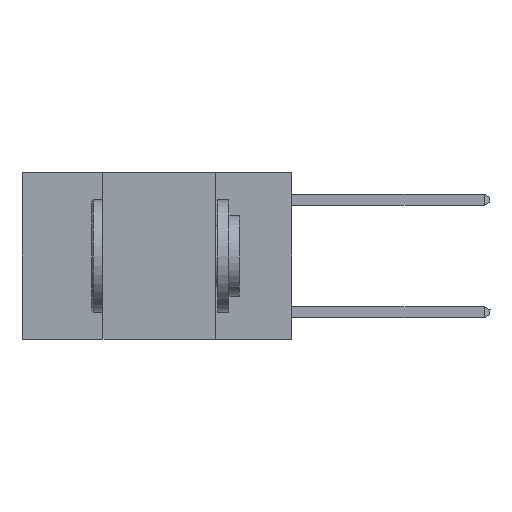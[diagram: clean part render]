
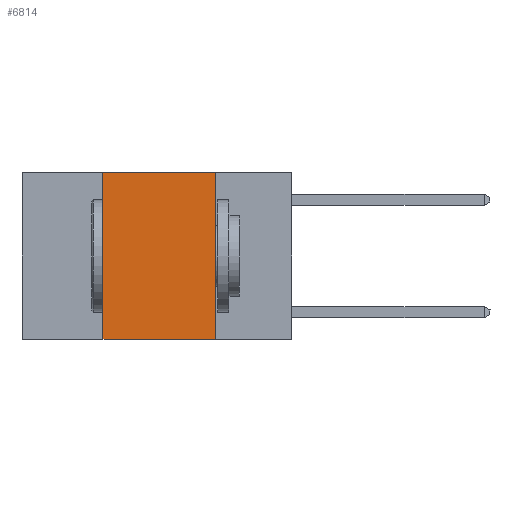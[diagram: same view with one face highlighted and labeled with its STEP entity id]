
A CAD part, left-side view. The second image highlights one B-rep face of the part: STEP entity #6814.
In plain terms, the highlighted planar face has unit normal (-1, 0, 0).
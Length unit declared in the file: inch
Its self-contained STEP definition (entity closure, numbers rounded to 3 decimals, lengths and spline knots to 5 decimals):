
#841 = VECTOR ( 'NONE', #13239, 39.37008 ) ;
#1133 = CARTESIAN_POINT ( 'NONE',  ( 0., 0.6, 0. ) ) ;
#1365 = DIRECTION ( 'NONE',  ( 0., 0., -1. ) ) ;
#2137 = CARTESIAN_POINT ( 'NONE',  ( 0., 0.42, -0.37 ) ) ;
#2207 = LINE ( 'NONE', #11647, #7037 ) ;
#3255 = DIRECTION ( 'NONE',  ( 1., 0., 0. ) ) ;
#4270 = LINE ( 'NONE', #20502, #19814 ) ;
#4390 = DIRECTION ( 'NONE',  ( 0., 0., 1. ) ) ;
#5343 = EDGE_CURVE ( 'NONE', #6308, #20521, #22432, .T. ) ;
#6036 = CARTESIAN_POINT ( 'NONE',  ( 0., 0.17, 0. ) ) ;
#6308 = VERTEX_POINT ( 'NONE', #19988 ) ;
#6814 = ADVANCED_FACE ( 'NONE', ( #22986 ), #15537, .F. ) ;
#7037 = VECTOR ( 'NONE', #1365, 39.37008 ) ;
#8282 = AXIS2_PLACEMENT_3D ( 'NONE', #1133, #3255, #17503 ) ;
#8550 = ORIENTED_EDGE ( 'NONE', *, *, #22767, .F. ) ;
#8698 = VERTEX_POINT ( 'NONE', #15219 ) ;
#8865 = EDGE_CURVE ( 'NONE', #20521, #8698, #2207, .T. ) ;
#11647 = CARTESIAN_POINT ( 'NONE',  ( 0., 0.17, 0. ) ) ;
#13133 = ORIENTED_EDGE ( 'NONE', *, *, #18073, .T. ) ;
#13239 = DIRECTION ( 'NONE',  ( 0., -1., 0. ) ) ;
#14968 = EDGE_LOOP ( 'NONE', ( #21974, #25986, #8550, #13133 ) ) ;
#15219 = CARTESIAN_POINT ( 'NONE',  ( 0., 0.17, -0.37 ) ) ;
#15537 = PLANE ( 'NONE',  #8282 ) ;
#16527 = VECTOR ( 'NONE', #23500, 39.37008 ) ;
#17503 = DIRECTION ( 'NONE',  ( 0., 0., -1. ) ) ;
#18073 = EDGE_CURVE ( 'NONE', #25201, #8698, #22391, .T. ) ;
#19814 = VECTOR ( 'NONE', #4390, 39.37008 ) ;
#19988 = CARTESIAN_POINT ( 'NONE',  ( 0., 0.42, 0. ) ) ;
#20502 = CARTESIAN_POINT ( 'NONE',  ( 0., 0.42, 0. ) ) ;
#20521 = VERTEX_POINT ( 'NONE', #6036 ) ;
#21171 = CARTESIAN_POINT ( 'NONE',  ( 0., 0.6, 0. ) ) ;
#21532 = CARTESIAN_POINT ( 'NONE',  ( 0., 0.6, -0.37 ) ) ;
#21974 = ORIENTED_EDGE ( 'NONE', *, *, #8865, .F. ) ;
#22391 = LINE ( 'NONE', #21532, #16527 ) ;
#22432 = LINE ( 'NONE', #21171, #841 ) ;
#22767 = EDGE_CURVE ( 'NONE', #25201, #6308, #4270, .T. ) ;
#22986 = FACE_OUTER_BOUND ( 'NONE', #14968, .T. ) ;
#23500 = DIRECTION ( 'NONE',  ( 0., -1., 0. ) ) ;
#25201 = VERTEX_POINT ( 'NONE', #2137 ) ;
#25986 = ORIENTED_EDGE ( 'NONE', *, *, #5343, .F. ) ;
